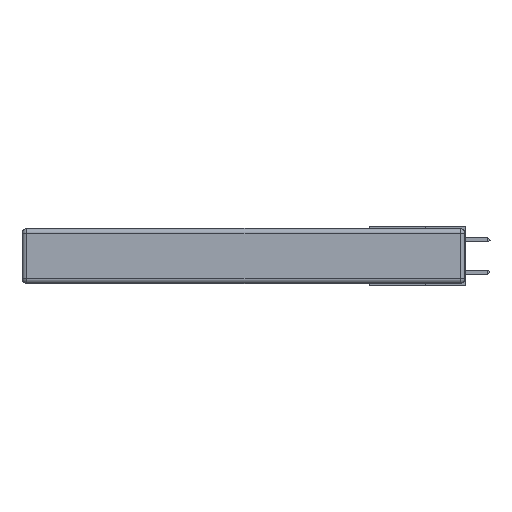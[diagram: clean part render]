
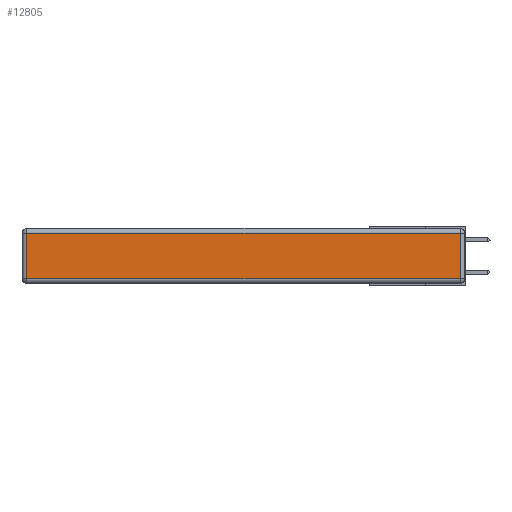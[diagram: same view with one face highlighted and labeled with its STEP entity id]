
A CAD part, left-side view. The second image highlights one B-rep face of the part: STEP entity #12805.
In plain terms, the highlighted planar face has unit normal (-1, 0, 0).
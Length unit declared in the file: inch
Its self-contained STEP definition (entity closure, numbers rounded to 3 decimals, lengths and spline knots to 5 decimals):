
#1331 = DIRECTION ( 'NONE',  ( 0., 0., -1. ) ) ;
#1372 = ORIENTED_EDGE ( 'NONE', *, *, #14798, .T. ) ;
#2147 = CARTESIAN_POINT ( 'NONE',  ( 0., 0., -0.313 ) ) ;
#2606 = VECTOR ( 'NONE', #15637, 39.37008 ) ;
#2763 = VERTEX_POINT ( 'NONE', #23025 ) ;
#2930 = ORIENTED_EDGE ( 'NONE', *, *, #16408, .T. ) ;
#3301 = EDGE_CURVE ( 'NONE', #2763, #20749, #7409, .T. ) ;
#4634 = DIRECTION ( 'NONE',  ( 0., 0., 1. ) ) ;
#5438 = ORIENTED_EDGE ( 'NONE', *, *, #3301, .T. ) ;
#5937 = VECTOR ( 'NONE', #20434, 39.37008 ) ;
#7028 = LINE ( 'NONE', #22478, #24295 ) ;
#7322 = CARTESIAN_POINT ( 'NONE',  ( 0., 2.72, -0.03 ) ) ;
#7409 = LINE ( 'NONE', #2147, #2606 ) ;
#12388 = DIRECTION ( 'NONE',  ( 0., 0., 1. ) ) ;
#12420 = ORIENTED_EDGE ( 'NONE', *, *, #20720, .T. ) ;
#12785 = VERTEX_POINT ( 'NONE', #23999 ) ;
#12805 = ADVANCED_FACE ( 'NONE', ( #23002 ), #18324, .T. ) ;
#13048 = EDGE_LOOP ( 'NONE', ( #5438, #12420, #1372, #2930 ) ) ;
#14798 = EDGE_CURVE ( 'NONE', #12785, #17160, #18322, .T. ) ;
#15637 = DIRECTION ( 'NONE',  ( 0., -1., 0. ) ) ;
#16297 = DIRECTION ( 'NONE',  ( -1., 0., 0. ) ) ;
#16408 = EDGE_CURVE ( 'NONE', #17160, #2763, #7028, .T. ) ;
#17160 = VERTEX_POINT ( 'NONE', #7322 ) ;
#17487 = VECTOR ( 'NONE', #12388, 39.37008 ) ;
#17966 = CARTESIAN_POINT ( 'NONE',  ( 0., 0.03, -0.313 ) ) ;
#18322 = LINE ( 'NONE', #22313, #5937 ) ;
#18324 = PLANE ( 'NONE',  #20345 ) ;
#19285 = LINE ( 'NONE', #22071, #17487 ) ;
#20205 = CARTESIAN_POINT ( 'NONE',  ( 0., 0., -0.343 ) ) ;
#20345 = AXIS2_PLACEMENT_3D ( 'NONE', #20205, #16297, #4634 ) ;
#20434 = DIRECTION ( 'NONE',  ( 0., 1., 0. ) ) ;
#20720 = EDGE_CURVE ( 'NONE', #20749, #12785, #19285, .T. ) ;
#20749 = VERTEX_POINT ( 'NONE', #17966 ) ;
#22071 = CARTESIAN_POINT ( 'NONE',  ( 0., 0.03, -0.343 ) ) ;
#22313 = CARTESIAN_POINT ( 'NONE',  ( 0., 2.75, -0.03 ) ) ;
#22478 = CARTESIAN_POINT ( 'NONE',  ( 0., 2.72, -0.343 ) ) ;
#23002 = FACE_OUTER_BOUND ( 'NONE', #13048, .T. ) ;
#23025 = CARTESIAN_POINT ( 'NONE',  ( 0., 2.72, -0.313 ) ) ;
#23999 = CARTESIAN_POINT ( 'NONE',  ( 0., 0.03, -0.03 ) ) ;
#24295 = VECTOR ( 'NONE', #1331, 39.37008 ) ;
